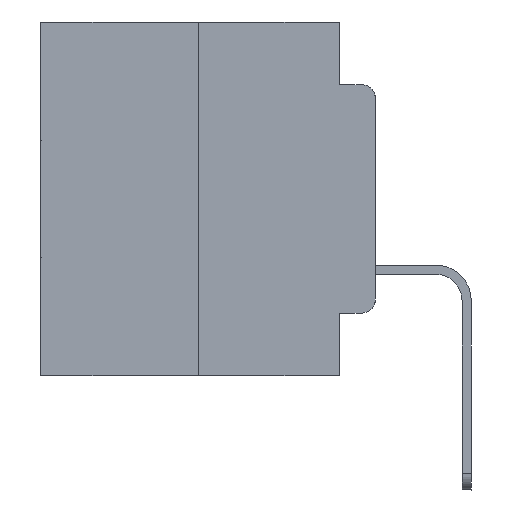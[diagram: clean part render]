
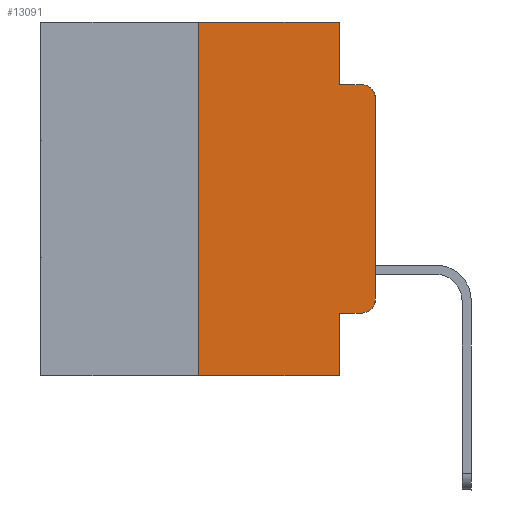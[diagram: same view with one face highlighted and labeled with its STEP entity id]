
A CAD part, left-side view. The second image highlights one B-rep face of the part: STEP entity #13091.
In plain terms, the highlighted planar face has unit normal (-1, 0, 0).
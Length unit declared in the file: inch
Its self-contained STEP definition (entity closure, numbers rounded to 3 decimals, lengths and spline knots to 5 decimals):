
#964 = EDGE_CURVE ( 'NONE', #2267, #6751, #19225, .T. ) ;
#1036 = AXIS2_PLACEMENT_3D ( 'NONE', #18359, #3973, #14218 ) ;
#1616 = CARTESIAN_POINT ( 'NONE',  ( 0., 0., -0.1085 ) ) ;
#1972 = EDGE_CURVE ( 'NONE', #11380, #19997, #10816, .T. ) ;
#2048 = DIRECTION ( 'NONE',  ( 0., 0., -1. ) ) ;
#2219 = LINE ( 'NONE', #17442, #15739 ) ;
#2267 = VERTEX_POINT ( 'NONE', #4875 ) ;
#2924 = EDGE_CURVE ( 'NONE', #3079, #18320, #15586, .T. ) ;
#2963 = LINE ( 'NONE', #19949, #10643 ) ;
#3057 = DIRECTION ( 'NONE',  ( 0., -1., 0. ) ) ;
#3079 = VERTEX_POINT ( 'NONE', #24040 ) ;
#3401 = DIRECTION ( 'NONE',  ( 0., 0., 1. ) ) ;
#3790 = AXIS2_PLACEMENT_3D ( 'NONE', #7907, #5940, #2048 ) ;
#3973 = DIRECTION ( 'NONE',  ( -1., 0., 0. ) ) ;
#4472 = EDGE_CURVE ( 'NONE', #19997, #6238, #2963, .T. ) ;
#4875 = CARTESIAN_POINT ( 'NONE',  ( 0., 0.25, -0.5 ) ) ;
#5051 = CARTESIAN_POINT ( 'NONE',  ( 0., 0.02, -0.4115 ) ) ;
#5940 = DIRECTION ( 'NONE',  ( -1., 0., 0. ) ) ;
#6133 = ORIENTED_EDGE ( 'NONE', *, *, #17842, .F. ) ;
#6238 = VERTEX_POINT ( 'NONE', #1616 ) ;
#6393 = CARTESIAN_POINT ( 'NONE',  ( 0., 0.051, 0. ) ) ;
#6403 = EDGE_CURVE ( 'NONE', #6238, #15537, #19250, .T. ) ;
#6751 = VERTEX_POINT ( 'NONE', #11112 ) ;
#7307 = CARTESIAN_POINT ( 'NONE',  ( 0., 0.473, 0. ) ) ;
#7362 = CARTESIAN_POINT ( 'NONE',  ( 0., 0.473, 0. ) ) ;
#7489 = VECTOR ( 'NONE', #11474, 39.37008 ) ;
#7626 = EDGE_CURVE ( 'NONE', #13139, #8253, #22748, .T. ) ;
#7651 = VECTOR ( 'NONE', #14266, 39.37008 ) ;
#7907 = CARTESIAN_POINT ( 'NONE',  ( 0., 0.02, -0.1085 ) ) ;
#7926 = CARTESIAN_POINT ( 'NONE',  ( 0., 0., -0.3915 ) ) ;
#8253 = VERTEX_POINT ( 'NONE', #21215 ) ;
#8647 = CARTESIAN_POINT ( 'NONE',  ( 0., 0.051, -0.4115 ) ) ;
#8866 = ORIENTED_EDGE ( 'NONE', *, *, #15444, .F. ) ;
#9228 = VECTOR ( 'NONE', #14572, 39.37008 ) ;
#9963 = CARTESIAN_POINT ( 'NONE',  ( 0., 0.473, -0.5 ) ) ;
#10126 = CARTESIAN_POINT ( 'NONE',  ( 0., 0.25, 0. ) ) ;
#10482 = LINE ( 'NONE', #14745, #9228 ) ;
#10643 = VECTOR ( 'NONE', #3401, 39.37008 ) ;
#10685 = DIRECTION ( 'NONE',  ( 1., 0., 0. ) ) ;
#10758 = CARTESIAN_POINT ( 'NONE',  ( 0., 0.02, -0.0885 ) ) ;
#10816 = CIRCLE ( 'NONE', #1036, 0.02 ) ;
#11112 = CARTESIAN_POINT ( 'NONE',  ( 0., 0.25, 0. ) ) ;
#11281 = DIRECTION ( 'NONE',  ( 0., 0., -1. ) ) ;
#11380 = VERTEX_POINT ( 'NONE', #5051 ) ;
#11474 = DIRECTION ( 'NONE',  ( 0., -1., 0. ) ) ;
#11623 = ORIENTED_EDGE ( 'NONE', *, *, #23653, .T. ) ;
#11836 = ORIENTED_EDGE ( 'NONE', *, *, #964, .F. ) ;
#13091 = ADVANCED_FACE ( 'NONE', ( #15861 ), #16903, .F. ) ;
#13139 = VERTEX_POINT ( 'NONE', #8647 ) ;
#13870 = EDGE_CURVE ( 'NONE', #13139, #11380, #2219, .T. ) ;
#14218 = DIRECTION ( 'NONE',  ( 0., 0., -1. ) ) ;
#14266 = DIRECTION ( 'NONE',  ( 0., 0., 1. ) ) ;
#14572 = DIRECTION ( 'NONE',  ( 0., -1., 0. ) ) ;
#14745 = CARTESIAN_POINT ( 'NONE',  ( 0., 0.051, -0.0885 ) ) ;
#15349 = CARTESIAN_POINT ( 'NONE',  ( 0., 0.051, -0.0885 ) ) ;
#15444 = EDGE_CURVE ( 'NONE', #18320, #15537, #10482, .T. ) ;
#15537 = VERTEX_POINT ( 'NONE', #10758 ) ;
#15586 = LINE ( 'NONE', #17236, #19131 ) ;
#15739 = VECTOR ( 'NONE', #3057, 39.37008 ) ;
#15861 = FACE_OUTER_BOUND ( 'NONE', #23072, .T. ) ;
#16607 = ORIENTED_EDGE ( 'NONE', *, *, #2924, .F. ) ;
#16903 = PLANE ( 'NONE',  #26412 ) ;
#17086 = ORIENTED_EDGE ( 'NONE', *, *, #6403, .T. ) ;
#17236 = CARTESIAN_POINT ( 'NONE',  ( 0., 0.051, 0. ) ) ;
#17442 = CARTESIAN_POINT ( 'NONE',  ( 0., 0.051, -0.4115 ) ) ;
#17842 = EDGE_CURVE ( 'NONE', #6751, #3079, #20337, .T. ) ;
#17950 = VECTOR ( 'NONE', #25047, 39.37008 ) ;
#18320 = VERTEX_POINT ( 'NONE', #15349 ) ;
#18359 = CARTESIAN_POINT ( 'NONE',  ( 0., 0.02, -0.3915 ) ) ;
#19039 = LINE ( 'NONE', #9963, #23191 ) ;
#19131 = VECTOR ( 'NONE', #11281, 39.37008 ) ;
#19225 = LINE ( 'NONE', #10126, #7651 ) ;
#19250 = CIRCLE ( 'NONE', #3790, 0.02 ) ;
#19763 = ORIENTED_EDGE ( 'NONE', *, *, #4472, .T. ) ;
#19949 = CARTESIAN_POINT ( 'NONE',  ( 0., 0., 0. ) ) ;
#19997 = VERTEX_POINT ( 'NONE', #7926 ) ;
#20337 = LINE ( 'NONE', #7362, #7489 ) ;
#20565 = ORIENTED_EDGE ( 'NONE', *, *, #13870, .T. ) ;
#21215 = CARTESIAN_POINT ( 'NONE',  ( 0., 0.051, -0.5 ) ) ;
#21692 = ORIENTED_EDGE ( 'NONE', *, *, #7626, .F. ) ;
#22748 = LINE ( 'NONE', #6393, #17950 ) ;
#23072 = EDGE_LOOP ( 'NONE', ( #19763, #17086, #8866, #16607, #6133, #11836, #11623, #21692, #20565, #24651 ) ) ;
#23180 = DIRECTION ( 'NONE',  ( 0., 0., -1. ) ) ;
#23191 = VECTOR ( 'NONE', #24409, 39.37008 ) ;
#23653 = EDGE_CURVE ( 'NONE', #2267, #8253, #19039, .T. ) ;
#24040 = CARTESIAN_POINT ( 'NONE',  ( 0., 0.051, 0. ) ) ;
#24409 = DIRECTION ( 'NONE',  ( 0., -1., 0. ) ) ;
#24651 = ORIENTED_EDGE ( 'NONE', *, *, #1972, .T. ) ;
#25047 = DIRECTION ( 'NONE',  ( 0., 0., -1. ) ) ;
#26412 = AXIS2_PLACEMENT_3D ( 'NONE', #7307, #10685, #23180 ) ;
